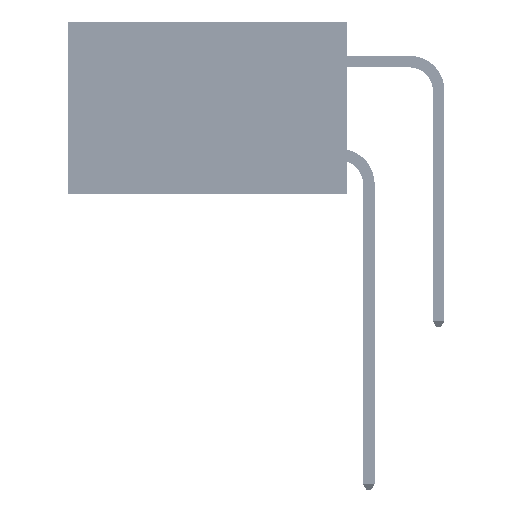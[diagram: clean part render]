
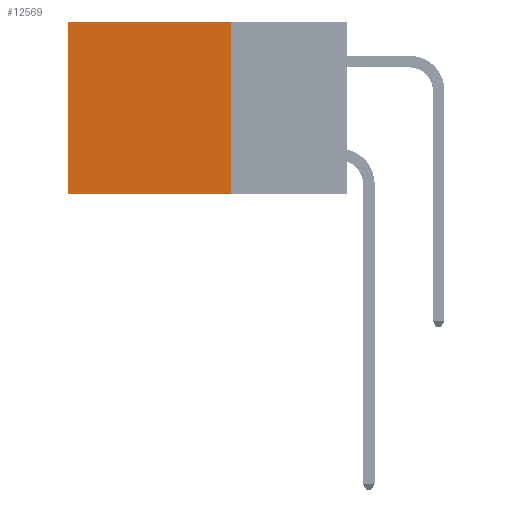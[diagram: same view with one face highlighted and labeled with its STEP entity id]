
A CAD part, left-side view. The second image highlights one B-rep face of the part: STEP entity #12569.
In plain terms, the highlighted planar face has unit normal (-1, 0, 0).
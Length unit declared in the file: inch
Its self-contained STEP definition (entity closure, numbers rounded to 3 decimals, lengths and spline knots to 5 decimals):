
#4142 = VERTEX_POINT ( 'NONE', #37493 ) ;
#6587 = ORIENTED_EDGE ( 'NONE', *, *, #41956, .F. ) ;
#6737 = EDGE_CURVE ( 'NONE', #4142, #19122, #20100, .T. ) ;
#7728 = DIRECTION ( 'NONE',  ( 0., 1., 0. ) ) ;
#8275 = LINE ( 'NONE', #31115, #22811 ) ;
#9123 = LINE ( 'NONE', #30953, #38809 ) ;
#9518 = CARTESIAN_POINT ( 'NONE',  ( 0.2875, 0.6, 0. ) ) ;
#10149 = ORIENTED_EDGE ( 'NONE', *, *, #6737, .T. ) ;
#12569 = ADVANCED_FACE ( 'NONE', ( #35300 ), #40141, .F. ) ;
#13485 = CARTESIAN_POINT ( 'NONE',  ( 0.2875, 0.6, 0. ) ) ;
#13719 = ORIENTED_EDGE ( 'NONE', *, *, #15374, .F. ) ;
#15374 = EDGE_CURVE ( 'NONE', #4142, #24021, #9123, .T. ) ;
#15520 = DIRECTION ( 'NONE',  ( 0., 0., -1. ) ) ;
#15870 = VERTEX_POINT ( 'NONE', #45017 ) ;
#15943 = LINE ( 'NONE', #13485, #34800 ) ;
#16949 = DIRECTION ( 'NONE',  ( 1., 0., 0. ) ) ;
#19122 = VERTEX_POINT ( 'NONE', #9518 ) ;
#19603 = DIRECTION ( 'NONE',  ( 0., 1., 0. ) ) ;
#20100 = LINE ( 'NONE', #27167, #39496 ) ;
#20804 = DIRECTION ( 'NONE',  ( 0., 0., -1. ) ) ;
#22811 = VECTOR ( 'NONE', #19603, 39.37008 ) ;
#24021 = VERTEX_POINT ( 'NONE', #25747 ) ;
#25747 = CARTESIAN_POINT ( 'NONE',  ( 0.2875, 0.25, -0.37 ) ) ;
#27167 = CARTESIAN_POINT ( 'NONE',  ( 0.2875, 0.25, 0. ) ) ;
#30953 = CARTESIAN_POINT ( 'NONE',  ( 0.2875, 0.25, 0. ) ) ;
#31115 = CARTESIAN_POINT ( 'NONE',  ( 0.2875, 0.25, -0.37 ) ) ;
#34619 = ORIENTED_EDGE ( 'NONE', *, *, #44280, .T. ) ;
#34800 = VECTOR ( 'NONE', #36890, 39.37008 ) ;
#35300 = FACE_OUTER_BOUND ( 'NONE', #36236, .T. ) ;
#35931 = CARTESIAN_POINT ( 'NONE',  ( 0.2875, 0.25, 0. ) ) ;
#36236 = EDGE_LOOP ( 'NONE', ( #34619, #6587, #13719, #10149 ) ) ;
#36890 = DIRECTION ( 'NONE',  ( 0., 0., -1. ) ) ;
#37493 = CARTESIAN_POINT ( 'NONE',  ( 0.2875, 0.25, 0. ) ) ;
#38809 = VECTOR ( 'NONE', #15520, 39.37008 ) ;
#39496 = VECTOR ( 'NONE', #7728, 39.37008 ) ;
#40141 = PLANE ( 'NONE',  #43661 ) ;
#41956 = EDGE_CURVE ( 'NONE', #24021, #15870, #8275, .T. ) ;
#43661 = AXIS2_PLACEMENT_3D ( 'NONE', #35931, #16949, #20804 ) ;
#44280 = EDGE_CURVE ( 'NONE', #19122, #15870, #15943, .T. ) ;
#45017 = CARTESIAN_POINT ( 'NONE',  ( 0.2875, 0.6, -0.37 ) ) ;
